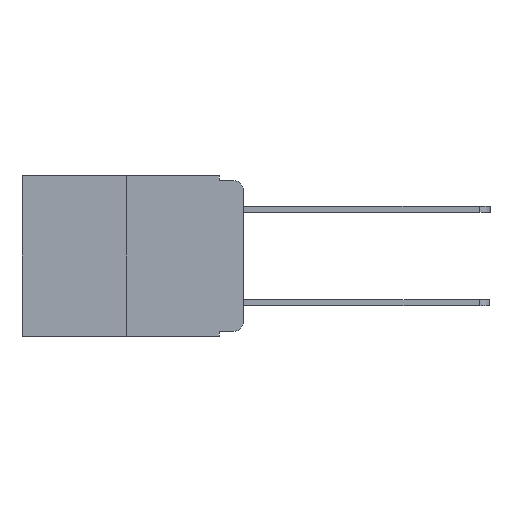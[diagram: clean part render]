
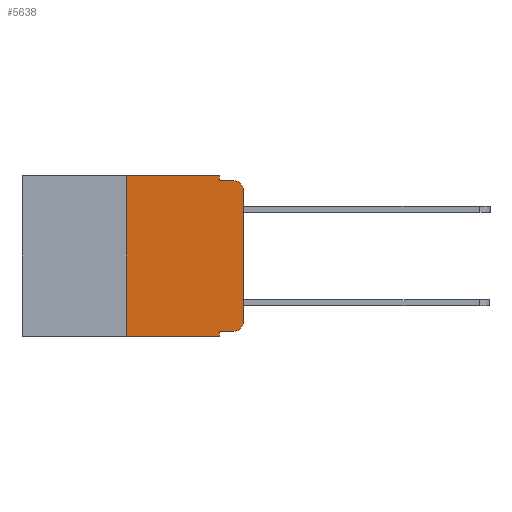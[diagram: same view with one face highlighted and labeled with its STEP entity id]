
A CAD part, left-side view. The second image highlights one B-rep face of the part: STEP entity #5638.
In plain terms, the highlighted planar face has unit normal (-1, 0, 0).
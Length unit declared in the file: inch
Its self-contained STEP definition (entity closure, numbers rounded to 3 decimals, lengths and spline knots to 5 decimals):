
#139 = CARTESIAN_POINT ( 'NONE',  ( 0., 0.473, 0. ) ) ;
#147 = VECTOR ( 'NONE', #1028, 39.37008 ) ;
#730 = DIRECTION ( 'NONE',  ( 1., 0., 0. ) ) ;
#770 = ORIENTED_EDGE ( 'NONE', *, *, #9507, .T. ) ;
#1028 = DIRECTION ( 'NONE',  ( 0., 0., -1. ) ) ;
#1461 = AXIS2_PLACEMENT_3D ( 'NONE', #8534, #2950, #9449 ) ;
#1884 = LINE ( 'NONE', #4238, #9072 ) ;
#2042 = DIRECTION ( 'NONE',  ( 0., -1., 0. ) ) ;
#2261 = ORIENTED_EDGE ( 'NONE', *, *, #8580, .T. ) ;
#2369 = ORIENTED_EDGE ( 'NONE', *, *, #10166, .F. ) ;
#2482 = DIRECTION ( 'NONE',  ( 0., -1., 0. ) ) ;
#2559 = VERTEX_POINT ( 'NONE', #11978 ) ;
#2699 = CARTESIAN_POINT ( 'NONE',  ( 0., 0.02, -0.03 ) ) ;
#2950 = DIRECTION ( 'NONE',  ( -1., 0., 0. ) ) ;
#3060 = VERTEX_POINT ( 'NONE', #5246 ) ;
#3085 = CARTESIAN_POINT ( 'NONE',  ( 0., 0.02, -0.01 ) ) ;
#3148 = EDGE_CURVE ( 'NONE', #8370, #8532, #3900, .T. ) ;
#3342 = ORIENTED_EDGE ( 'NONE', *, *, #8818, .F. ) ;
#3476 = CARTESIAN_POINT ( 'NONE',  ( 0., 0.051, 0. ) ) ;
#3607 = CARTESIAN_POINT ( 'NONE',  ( 0., 0.473, 0. ) ) ;
#3628 = LINE ( 'NONE', #9867, #6180 ) ;
#3636 = DIRECTION ( 'NONE',  ( 0., 0., -1. ) ) ;
#3666 = EDGE_CURVE ( 'NONE', #5380, #6130, #1884, .T. ) ;
#3881 = CARTESIAN_POINT ( 'NONE',  ( 0., 0.051, 0. ) ) ;
#3900 = LINE ( 'NONE', #3476, #10921 ) ;
#4080 = CARTESIAN_POINT ( 'NONE',  ( 0., 0.25, -0.343 ) ) ;
#4102 = VECTOR ( 'NONE', #2482, 39.37008 ) ;
#4238 = CARTESIAN_POINT ( 'NONE',  ( 0., 0.25, 0. ) ) ;
#4284 = LINE ( 'NONE', #139, #6840 ) ;
#4703 = VERTEX_POINT ( 'NONE', #3085 ) ;
#4993 = CIRCLE ( 'NONE', #1461, 0.02 ) ;
#5020 = CARTESIAN_POINT ( 'NONE',  ( 0., 0.051, -0.333 ) ) ;
#5246 = CARTESIAN_POINT ( 'NONE',  ( 0., 0., -0.03 ) ) ;
#5254 = EDGE_CURVE ( 'NONE', #6262, #7579, #5304, .T. ) ;
#5304 = LINE ( 'NONE', #3881, #147 ) ;
#5380 = VERTEX_POINT ( 'NONE', #4080 ) ;
#5393 = CARTESIAN_POINT ( 'NONE',  ( 0., 0.02, -0.333 ) ) ;
#5490 = CARTESIAN_POINT ( 'NONE',  ( 0., 0.051, -0.333 ) ) ;
#5585 = CARTESIAN_POINT ( 'NONE',  ( 0., 0.051, -0.343 ) ) ;
#5638 = ADVANCED_FACE ( 'NONE', ( #11229 ), #6495, .F. ) ;
#5811 = ORIENTED_EDGE ( 'NONE', *, *, #11699, .T. ) ;
#5942 = DIRECTION ( 'NONE',  ( 0., -1., 0. ) ) ;
#5984 = CARTESIAN_POINT ( 'NONE',  ( 0., 0.051, 0. ) ) ;
#6101 = ORIENTED_EDGE ( 'NONE', *, *, #11384, .T. ) ;
#6130 = VERTEX_POINT ( 'NONE', #6241 ) ;
#6180 = VECTOR ( 'NONE', #8081, 39.37008 ) ;
#6241 = CARTESIAN_POINT ( 'NONE',  ( 0., 0.25, 0. ) ) ;
#6262 = VERTEX_POINT ( 'NONE', #5490 ) ;
#6495 = PLANE ( 'NONE',  #7567 ) ;
#6664 = ORIENTED_EDGE ( 'NONE', *, *, #5254, .F. ) ;
#6673 = LINE ( 'NONE', #8088, #4102 ) ;
#6840 = VECTOR ( 'NONE', #5942, 39.37008 ) ;
#6861 = VERTEX_POINT ( 'NONE', #5393 ) ;
#6943 = VECTOR ( 'NONE', #2042, 39.37008 ) ;
#6948 = DIRECTION ( 'NONE',  ( 0., 0., 1. ) ) ;
#7266 = CIRCLE ( 'NONE', #8929, 0.02 ) ;
#7320 = CARTESIAN_POINT ( 'NONE',  ( 0., 0.051, -0.01 ) ) ;
#7406 = DIRECTION ( 'NONE',  ( 0., 0., -1. ) ) ;
#7548 = ORIENTED_EDGE ( 'NONE', *, *, #3148, .F. ) ;
#7567 = AXIS2_PLACEMENT_3D ( 'NONE', #3607, #730, #7406 ) ;
#7579 = VERTEX_POINT ( 'NONE', #5585 ) ;
#7799 = ORIENTED_EDGE ( 'NONE', *, *, #10573, .T. ) ;
#8081 = DIRECTION ( 'NONE',  ( 0., -1., 0. ) ) ;
#8088 = CARTESIAN_POINT ( 'NONE',  ( 0., 0.051, -0.01 ) ) ;
#8370 = VERTEX_POINT ( 'NONE', #5984 ) ;
#8532 = VERTEX_POINT ( 'NONE', #7320 ) ;
#8534 = CARTESIAN_POINT ( 'NONE',  ( 0., 0.02, -0.313 ) ) ;
#8580 = EDGE_CURVE ( 'NONE', #3060, #4703, #7266, .T. ) ;
#8818 = EDGE_CURVE ( 'NONE', #6130, #8370, #4284, .T. ) ;
#8929 = AXIS2_PLACEMENT_3D ( 'NONE', #2699, #9195, #3636 ) ;
#8978 = ORIENTED_EDGE ( 'NONE', *, *, #3666, .F. ) ;
#9072 = VECTOR ( 'NONE', #10663, 39.37008 ) ;
#9195 = DIRECTION ( 'NONE',  ( -1., 0., 0. ) ) ;
#9206 = LINE ( 'NONE', #11378, #11280 ) ;
#9449 = DIRECTION ( 'NONE',  ( 0., 0., -1. ) ) ;
#9507 = EDGE_CURVE ( 'NONE', #2559, #3060, #9206, .T. ) ;
#9867 = CARTESIAN_POINT ( 'NONE',  ( 0., 0.473, -0.343 ) ) ;
#9894 = LINE ( 'NONE', #5020, #6943 ) ;
#9968 = DIRECTION ( 'NONE',  ( 0., 0., -1. ) ) ;
#10166 = EDGE_CURVE ( 'NONE', #8532, #4703, #6673, .T. ) ;
#10364 = EDGE_LOOP ( 'NONE', ( #770, #2261, #2369, #7548, #3342, #8978, #5811, #6664, #7799, #6101 ) ) ;
#10573 = EDGE_CURVE ( 'NONE', #6262, #6861, #9894, .T. ) ;
#10663 = DIRECTION ( 'NONE',  ( 0., 0., 1. ) ) ;
#10921 = VECTOR ( 'NONE', #9968, 39.37008 ) ;
#11229 = FACE_OUTER_BOUND ( 'NONE', #10364, .T. ) ;
#11280 = VECTOR ( 'NONE', #6948, 39.37008 ) ;
#11378 = CARTESIAN_POINT ( 'NONE',  ( 0., 0., 0. ) ) ;
#11384 = EDGE_CURVE ( 'NONE', #6861, #2559, #4993, .T. ) ;
#11699 = EDGE_CURVE ( 'NONE', #5380, #7579, #3628, .T. ) ;
#11978 = CARTESIAN_POINT ( 'NONE',  ( 0., 0., -0.313 ) ) ;
